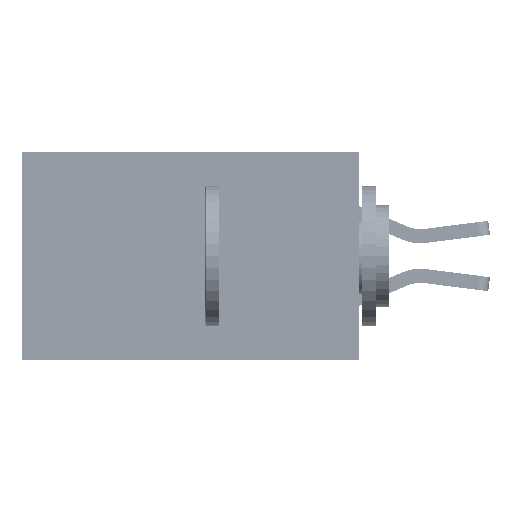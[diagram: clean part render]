
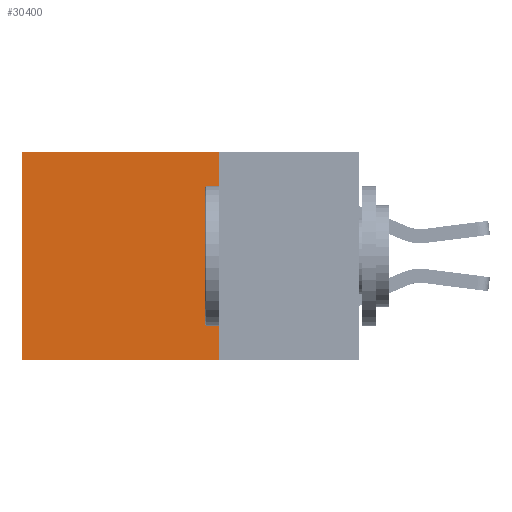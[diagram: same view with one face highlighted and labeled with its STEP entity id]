
A CAD part, left-side view. The second image highlights one B-rep face of the part: STEP entity #30400.
In plain terms, the highlighted planar face has unit normal (-1, 0, 0).
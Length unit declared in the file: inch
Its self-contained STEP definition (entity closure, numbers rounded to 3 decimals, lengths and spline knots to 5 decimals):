
#215 = EDGE_CURVE ( 'NONE', #24187, #9657, #7026, .T. ) ;
#506 = EDGE_CURVE ( 'NONE', #24187, #38605, #39369, .T. ) ;
#1009 = AXIS2_PLACEMENT_3D ( 'NONE', #9965, #2930, #35587 ) ;
#2821 = FACE_OUTER_BOUND ( 'NONE', #25966, .T. ) ;
#2930 = DIRECTION ( 'NONE',  ( 1., 0., 0. ) ) ;
#5774 = ORIENTED_EDGE ( 'NONE', *, *, #506, .F. ) ;
#5846 = EDGE_CURVE ( 'NONE', #9657, #39689, #17237, .T. ) ;
#6412 = VECTOR ( 'NONE', #17943, 39.37008 ) ;
#7026 = LINE ( 'NONE', #17885, #16003 ) ;
#9427 = DIRECTION ( 'NONE',  ( 0., 1., 0. ) ) ;
#9657 = VERTEX_POINT ( 'NONE', #20012 ) ;
#9965 = CARTESIAN_POINT ( 'NONE',  ( 0.2875, 0.25, 0. ) ) ;
#11265 = LINE ( 'NONE', #27100, #34781 ) ;
#13692 = CARTESIAN_POINT ( 'NONE',  ( 0.2875, 0.25, -0.37 ) ) ;
#16003 = VECTOR ( 'NONE', #25904, 39.37008 ) ;
#17237 = LINE ( 'NONE', #20474, #22279 ) ;
#17885 = CARTESIAN_POINT ( 'NONE',  ( 0.2875, 0.25, 0. ) ) ;
#17943 = DIRECTION ( 'NONE',  ( 0., 0., -1. ) ) ;
#20012 = CARTESIAN_POINT ( 'NONE',  ( 0.2875, 0.6, 0. ) ) ;
#20474 = CARTESIAN_POINT ( 'NONE',  ( 0.2875, 0.6, 0. ) ) ;
#22279 = VECTOR ( 'NONE', #38444, 39.37008 ) ;
#24187 = VERTEX_POINT ( 'NONE', #26741 ) ;
#24994 = PLANE ( 'NONE',  #1009 ) ;
#25904 = DIRECTION ( 'NONE',  ( 0., 1., 0. ) ) ;
#25966 = EDGE_LOOP ( 'NONE', ( #42550, #44246, #5774, #34974 ) ) ;
#26741 = CARTESIAN_POINT ( 'NONE',  ( 0.2875, 0.25, 0. ) ) ;
#27100 = CARTESIAN_POINT ( 'NONE',  ( 0.2875, 0.25, -0.37 ) ) ;
#27674 = CARTESIAN_POINT ( 'NONE',  ( 0.2875, 0.25, 0. ) ) ;
#29772 = EDGE_CURVE ( 'NONE', #38605, #39689, #11265, .T. ) ;
#30400 = ADVANCED_FACE ( 'NONE', ( #2821 ), #24994, .F. ) ;
#34781 = VECTOR ( 'NONE', #9427, 39.37008 ) ;
#34974 = ORIENTED_EDGE ( 'NONE', *, *, #215, .T. ) ;
#35587 = DIRECTION ( 'NONE',  ( 0., 0., -1. ) ) ;
#38444 = DIRECTION ( 'NONE',  ( 0., 0., -1. ) ) ;
#38605 = VERTEX_POINT ( 'NONE', #13692 ) ;
#39369 = LINE ( 'NONE', #27674, #6412 ) ;
#39689 = VERTEX_POINT ( 'NONE', #44425 ) ;
#42550 = ORIENTED_EDGE ( 'NONE', *, *, #5846, .T. ) ;
#44246 = ORIENTED_EDGE ( 'NONE', *, *, #29772, .F. ) ;
#44425 = CARTESIAN_POINT ( 'NONE',  ( 0.2875, 0.6, -0.37 ) ) ;
